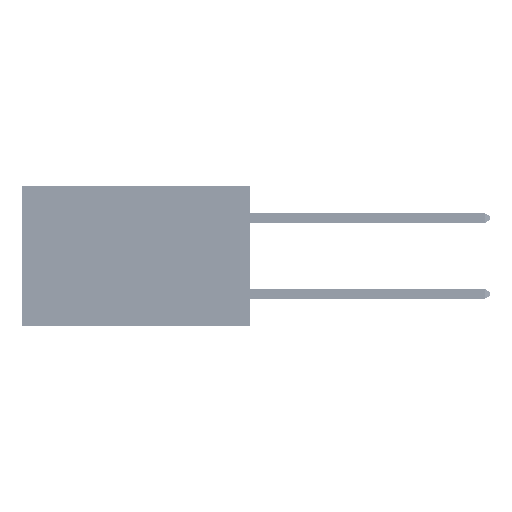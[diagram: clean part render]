
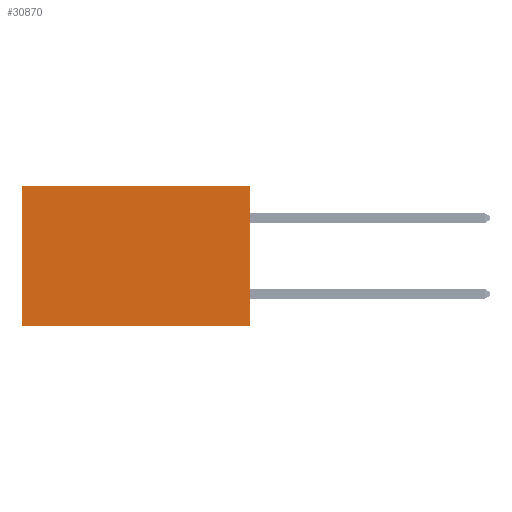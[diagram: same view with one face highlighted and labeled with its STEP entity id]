
A CAD part, left-side view. The second image highlights one B-rep face of the part: STEP entity #30870.
In plain terms, the highlighted planar face has unit normal (-1, 0, 0).
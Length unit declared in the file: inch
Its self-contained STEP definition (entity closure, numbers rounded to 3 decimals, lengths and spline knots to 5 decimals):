
#2818 = VECTOR ( 'NONE', #12719, 39.37008 ) ;
#4289 = ORIENTED_EDGE ( 'NONE', *, *, #8578, .F. ) ;
#6783 = CARTESIAN_POINT ( 'NONE',  ( 0.2875, 0., 0. ) ) ;
#8578 = EDGE_CURVE ( 'NONE', #37729, #20764, #21483, .T. ) ;
#10362 = DIRECTION ( 'NONE',  ( 1., 0., 0. ) ) ;
#12386 = FACE_OUTER_BOUND ( 'NONE', #34461, .T. ) ;
#12719 = DIRECTION ( 'NONE',  ( 0., 1., 0. ) ) ;
#13131 = VECTOR ( 'NONE', #39200, 39.37008 ) ;
#14535 = LINE ( 'NONE', #42508, #41392 ) ;
#15035 = ORIENTED_EDGE ( 'NONE', *, *, #46240, .F. ) ;
#16491 = CARTESIAN_POINT ( 'NONE',  ( 0.2875, 0., -0.37 ) ) ;
#17046 = CARTESIAN_POINT ( 'NONE',  ( 0.2875, 0.6, -0.37 ) ) ;
#17747 = EDGE_CURVE ( 'NONE', #30132, #20764, #40595, .T. ) ;
#18394 = CARTESIAN_POINT ( 'NONE',  ( 0.2875, 0., 0. ) ) ;
#19748 = CARTESIAN_POINT ( 'NONE',  ( 0.2875, 0.6, 0. ) ) ;
#20764 = VERTEX_POINT ( 'NONE', #17046 ) ;
#21483 = LINE ( 'NONE', #16491, #2818 ) ;
#22049 = VERTEX_POINT ( 'NONE', #27884 ) ;
#24512 = EDGE_CURVE ( 'NONE', #22049, #30132, #14535, .T. ) ;
#25068 = DIRECTION ( 'NONE',  ( 0., 0., -1. ) ) ;
#27884 = CARTESIAN_POINT ( 'NONE',  ( 0.2875, 0., 0. ) ) ;
#29093 = ORIENTED_EDGE ( 'NONE', *, *, #17747, .T. ) ;
#30132 = VERTEX_POINT ( 'NONE', #19748 ) ;
#30870 = ADVANCED_FACE ( 'NONE', ( #12386 ), #47597, .F. ) ;
#34428 = CARTESIAN_POINT ( 'NONE',  ( 0.2875, 0., -0.37 ) ) ;
#34461 = EDGE_LOOP ( 'NONE', ( #29093, #4289, #15035, #36844 ) ) ;
#36844 = ORIENTED_EDGE ( 'NONE', *, *, #24512, .T. ) ;
#37729 = VERTEX_POINT ( 'NONE', #34428 ) ;
#38062 = CARTESIAN_POINT ( 'NONE',  ( 0.2875, 0.6, 0. ) ) ;
#39061 = DIRECTION ( 'NONE',  ( 0., 1., 0. ) ) ;
#39200 = DIRECTION ( 'NONE',  ( 0., 0., -1. ) ) ;
#40220 = VECTOR ( 'NONE', #44476, 39.37008 ) ;
#40595 = LINE ( 'NONE', #38062, #13131 ) ;
#41392 = VECTOR ( 'NONE', #39061, 39.37008 ) ;
#42508 = CARTESIAN_POINT ( 'NONE',  ( 0.2875, 0., 0. ) ) ;
#43146 = LINE ( 'NONE', #18394, #40220 ) ;
#44476 = DIRECTION ( 'NONE',  ( 0., 0., -1. ) ) ;
#44739 = AXIS2_PLACEMENT_3D ( 'NONE', #6783, #10362, #25068 ) ;
#46240 = EDGE_CURVE ( 'NONE', #22049, #37729, #43146, .T. ) ;
#47597 = PLANE ( 'NONE',  #44739 ) ;
